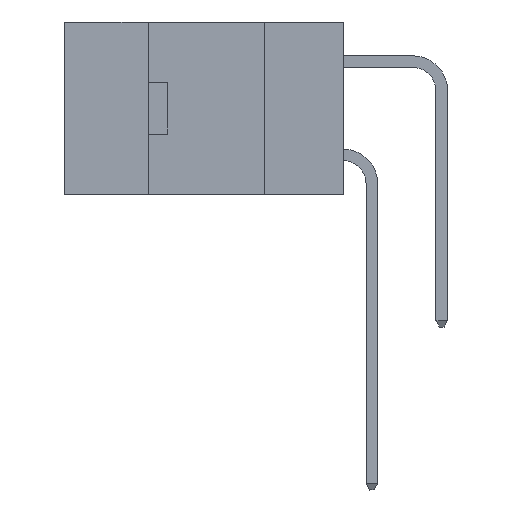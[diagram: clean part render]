
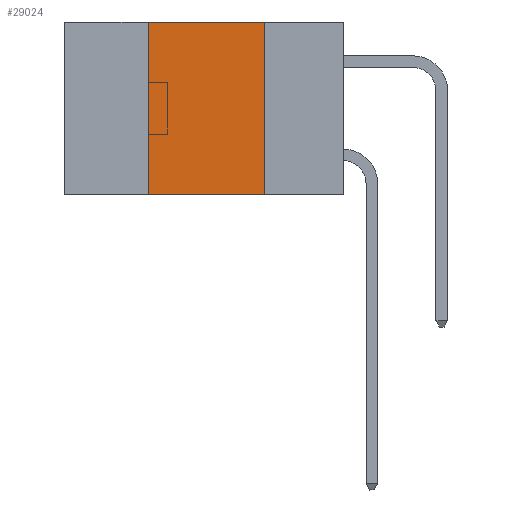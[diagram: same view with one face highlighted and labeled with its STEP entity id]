
A CAD part, left-side view. The second image highlights one B-rep face of the part: STEP entity #29024.
In plain terms, the highlighted planar face has unit normal (-1, 0, 0).
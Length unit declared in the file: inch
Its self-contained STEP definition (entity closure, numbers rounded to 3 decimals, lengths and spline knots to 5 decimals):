
#161 = CARTESIAN_POINT ( 'NONE',  ( 0., 0.42, -0.37 ) ) ;
#572 = CARTESIAN_POINT ( 'NONE',  ( 0., 0.17, -0.37 ) ) ;
#1613 = VECTOR ( 'NONE', #18186, 39.37008 ) ;
#1666 = DIRECTION ( 'NONE',  ( 0., -1., 0. ) ) ;
#1813 = VERTEX_POINT ( 'NONE', #10905 ) ;
#2118 = CARTESIAN_POINT ( 'NONE',  ( 0., 0.17, -0.37 ) ) ;
#2462 = VECTOR ( 'NONE', #1666, 39.37008 ) ;
#3282 = EDGE_LOOP ( 'NONE', ( #9707, #6766, #22619, #30506 ) ) ;
#4100 = EDGE_CURVE ( 'NONE', #11918, #14315, #6585, .T. ) ;
#4224 = CARTESIAN_POINT ( 'NONE',  ( 0., 0.42, 0. ) ) ;
#5741 = VECTOR ( 'NONE', #6594, 39.37008 ) ;
#6585 = LINE ( 'NONE', #15847, #1613 ) ;
#6594 = DIRECTION ( 'NONE',  ( 0., -1., 0. ) ) ;
#6766 = ORIENTED_EDGE ( 'NONE', *, *, #12345, .F. ) ;
#9338 = AXIS2_PLACEMENT_3D ( 'NONE', #20773, #25458, #11477 ) ;
#9544 = EDGE_CURVE ( 'NONE', #11918, #19938, #27638, .T. ) ;
#9707 = ORIENTED_EDGE ( 'NONE', *, *, #19010, .F. ) ;
#10905 = CARTESIAN_POINT ( 'NONE',  ( 0., 0.17, 0. ) ) ;
#11477 = DIRECTION ( 'NONE',  ( 0., 0., -1. ) ) ;
#11918 = VERTEX_POINT ( 'NONE', #161 ) ;
#12345 = EDGE_CURVE ( 'NONE', #14315, #1813, #30013, .T. ) ;
#14315 = VERTEX_POINT ( 'NONE', #4224 ) ;
#14859 = FACE_OUTER_BOUND ( 'NONE', #3282, .T. ) ;
#15847 = CARTESIAN_POINT ( 'NONE',  ( 0., 0.42, -0.37 ) ) ;
#18045 = LINE ( 'NONE', #572, #23509 ) ;
#18186 = DIRECTION ( 'NONE',  ( 0., 0., 1. ) ) ;
#19010 = EDGE_CURVE ( 'NONE', #1813, #19938, #18045, .T. ) ;
#19938 = VERTEX_POINT ( 'NONE', #2118 ) ;
#20773 = CARTESIAN_POINT ( 'NONE',  ( 0., 0.6, 0. ) ) ;
#21918 = DIRECTION ( 'NONE',  ( 0., 0., -1. ) ) ;
#22619 = ORIENTED_EDGE ( 'NONE', *, *, #4100, .F. ) ;
#23039 = CARTESIAN_POINT ( 'NONE',  ( 0., 0.6, 0. ) ) ;
#23125 = PLANE ( 'NONE',  #9338 ) ;
#23509 = VECTOR ( 'NONE', #21918, 39.37008 ) ;
#25288 = CARTESIAN_POINT ( 'NONE',  ( 0., 0.6, -0.37 ) ) ;
#25458 = DIRECTION ( 'NONE',  ( 1., 0., 0. ) ) ;
#27638 = LINE ( 'NONE', #25288, #2462 ) ;
#29024 = ADVANCED_FACE ( 'NONE', ( #14859 ), #23125, .F. ) ;
#30013 = LINE ( 'NONE', #23039, #5741 ) ;
#30506 = ORIENTED_EDGE ( 'NONE', *, *, #9544, .T. ) ;
